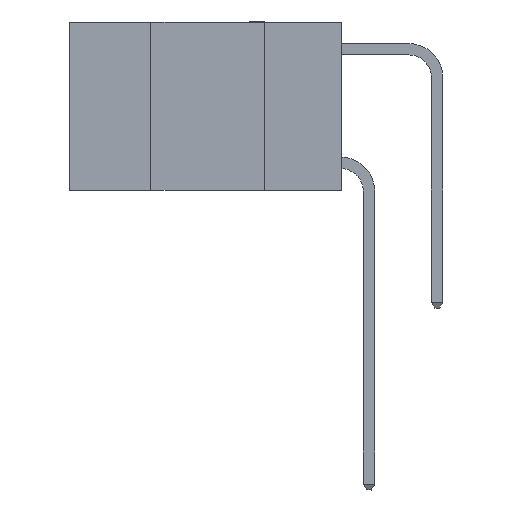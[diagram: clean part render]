
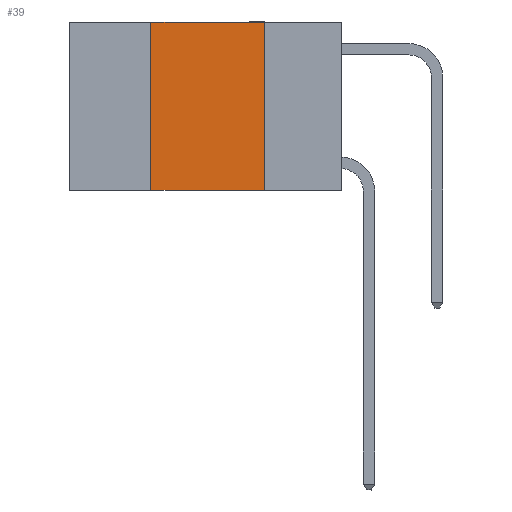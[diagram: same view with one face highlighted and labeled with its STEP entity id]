
A CAD part, left-side view. The second image highlights one B-rep face of the part: STEP entity #39.
In plain terms, the highlighted planar face has unit normal (-1, 0, 0).
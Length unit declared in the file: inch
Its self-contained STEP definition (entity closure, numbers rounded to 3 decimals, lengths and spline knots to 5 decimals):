
#39 = ADVANCED_FACE ( 'NONE', ( #11600 ), #5171, .F. ) ;
#399 = DIRECTION ( 'NONE',  ( 0., -1., 0. ) ) ;
#538 = VERTEX_POINT ( 'NONE', #7261 ) ;
#641 = EDGE_CURVE ( 'NONE', #5939, #7938, #15267, .T. ) ;
#657 = CARTESIAN_POINT ( 'NONE',  ( 0., 0.6, -0.37 ) ) ;
#684 = EDGE_LOOP ( 'NONE', ( #9310, #4983, #6049, #13266 ) ) ;
#3295 = CARTESIAN_POINT ( 'NONE',  ( 0., 0.6, 0. ) ) ;
#3564 = AXIS2_PLACEMENT_3D ( 'NONE', #3295, #15663, #14349 ) ;
#4983 = ORIENTED_EDGE ( 'NONE', *, *, #5272, .F. ) ;
#5171 = PLANE ( 'NONE',  #3564 ) ;
#5272 = EDGE_CURVE ( 'NONE', #15271, #538, #15729, .T. ) ;
#5409 = LINE ( 'NONE', #15293, #8895 ) ;
#5598 = CARTESIAN_POINT ( 'NONE',  ( 0., 0.17, 0. ) ) ;
#5939 = VERTEX_POINT ( 'NONE', #11775 ) ;
#6049 = ORIENTED_EDGE ( 'NONE', *, *, #12381, .F. ) ;
#6996 = CARTESIAN_POINT ( 'NONE',  ( 0., 0.42, 0. ) ) ;
#7261 = CARTESIAN_POINT ( 'NONE',  ( 0., 0.17, 0. ) ) ;
#7786 = CARTESIAN_POINT ( 'NONE',  ( 0., 0.17, -0.37 ) ) ;
#7938 = VERTEX_POINT ( 'NONE', #7786 ) ;
#8257 = EDGE_CURVE ( 'NONE', #538, #7938, #13809, .T. ) ;
#8836 = VECTOR ( 'NONE', #13262, 39.37008 ) ;
#8895 = VECTOR ( 'NONE', #11365, 39.37008 ) ;
#9310 = ORIENTED_EDGE ( 'NONE', *, *, #8257, .F. ) ;
#10371 = VECTOR ( 'NONE', #15944, 39.37008 ) ;
#11365 = DIRECTION ( 'NONE',  ( 0., 0., 1. ) ) ;
#11600 = FACE_OUTER_BOUND ( 'NONE', #684, .T. ) ;
#11775 = CARTESIAN_POINT ( 'NONE',  ( 0., 0.42, -0.37 ) ) ;
#12381 = EDGE_CURVE ( 'NONE', #5939, #15271, #5409, .T. ) ;
#12604 = VECTOR ( 'NONE', #399, 39.37008 ) ;
#13262 = DIRECTION ( 'NONE',  ( 0., -1., 0. ) ) ;
#13266 = ORIENTED_EDGE ( 'NONE', *, *, #641, .T. ) ;
#13809 = LINE ( 'NONE', #5598, #10371 ) ;
#14349 = DIRECTION ( 'NONE',  ( 0., 0., -1. ) ) ;
#14560 = CARTESIAN_POINT ( 'NONE',  ( 0., 0.6, 0. ) ) ;
#15267 = LINE ( 'NONE', #657, #12604 ) ;
#15271 = VERTEX_POINT ( 'NONE', #6996 ) ;
#15293 = CARTESIAN_POINT ( 'NONE',  ( 0., 0.42, 0. ) ) ;
#15663 = DIRECTION ( 'NONE',  ( 1., 0., 0. ) ) ;
#15729 = LINE ( 'NONE', #14560, #8836 ) ;
#15944 = DIRECTION ( 'NONE',  ( 0., 0., -1. ) ) ;
